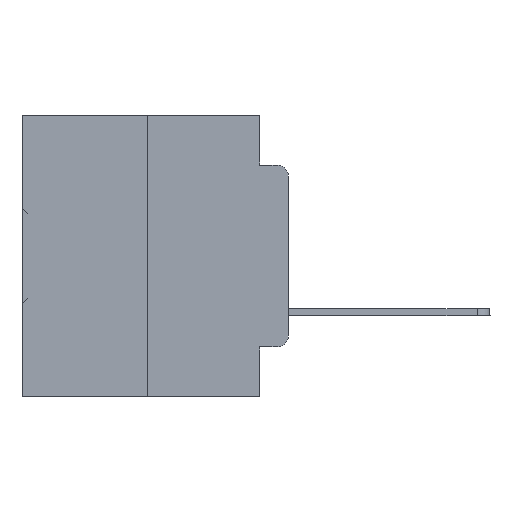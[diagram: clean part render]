
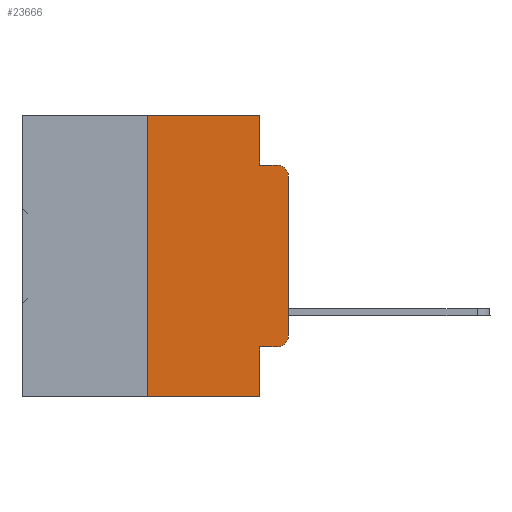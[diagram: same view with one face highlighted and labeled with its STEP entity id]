
A CAD part, left-side view. The second image highlights one B-rep face of the part: STEP entity #23666.
In plain terms, the highlighted planar face has unit normal (-1, 0, 0).
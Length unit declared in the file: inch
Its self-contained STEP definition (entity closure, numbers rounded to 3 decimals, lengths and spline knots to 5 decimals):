
#440 = CARTESIAN_POINT ( 'NONE',  ( 0., 0.25, 0. ) ) ;
#1844 = ORIENTED_EDGE ( 'NONE', *, *, #35728, .F. ) ;
#1858 = CARTESIAN_POINT ( 'NONE',  ( 0., 0.051, -0.0885 ) ) ;
#1861 = VERTEX_POINT ( 'NONE', #27456 ) ;
#2323 = CARTESIAN_POINT ( 'NONE',  ( 0., 0., -0.3915 ) ) ;
#2589 = DIRECTION ( 'NONE',  ( 0., 0., 1. ) ) ;
#2970 = EDGE_LOOP ( 'NONE', ( #31166, #35959, #24274, #21436, #34264, #14119, #27067, #1844, #8070, #9068 ) ) ;
#3821 = AXIS2_PLACEMENT_3D ( 'NONE', #16597, #28129, #8320 ) ;
#4102 = VECTOR ( 'NONE', #35673, 39.37008 ) ;
#4434 = EDGE_CURVE ( 'NONE', #31524, #20367, #23377, .T. ) ;
#4516 = FACE_OUTER_BOUND ( 'NONE', #2970, .T. ) ;
#4944 = CARTESIAN_POINT ( 'NONE',  ( 0., 0.051, -0.0885 ) ) ;
#4979 = AXIS2_PLACEMENT_3D ( 'NONE', #27903, #11076, #25078 ) ;
#5145 = VERTEX_POINT ( 'NONE', #29237 ) ;
#6379 = VERTEX_POINT ( 'NONE', #17656 ) ;
#6495 = LINE ( 'NONE', #20571, #27211 ) ;
#6740 = LINE ( 'NONE', #7071, #22135 ) ;
#7071 = CARTESIAN_POINT ( 'NONE',  ( 0., 0.051, 0. ) ) ;
#7100 = CARTESIAN_POINT ( 'NONE',  ( 0., 0.473, -0.5 ) ) ;
#8070 = ORIENTED_EDGE ( 'NONE', *, *, #13302, .T. ) ;
#8320 = DIRECTION ( 'NONE',  ( 0., 0., -1. ) ) ;
#9068 = ORIENTED_EDGE ( 'NONE', *, *, #19667, .T. ) ;
#9820 = LINE ( 'NONE', #29593, #4102 ) ;
#10162 = EDGE_CURVE ( 'NONE', #20367, #12212, #17248, .T. ) ;
#10170 = VECTOR ( 'NONE', #23088, 39.37008 ) ;
#10440 = EDGE_CURVE ( 'NONE', #30002, #5145, #31272, .T. ) ;
#10610 = CARTESIAN_POINT ( 'NONE',  ( 0., 0.051, 0. ) ) ;
#11076 = DIRECTION ( 'NONE',  ( -1., 0., 0. ) ) ;
#12212 = VERTEX_POINT ( 'NONE', #33256 ) ;
#12769 = DIRECTION ( 'NONE',  ( 0., -1., 0. ) ) ;
#13302 = EDGE_CURVE ( 'NONE', #1861, #6379, #6495, .T. ) ;
#13354 = DIRECTION ( 'NONE',  ( 0., 0., -1. ) ) ;
#13934 = AXIS2_PLACEMENT_3D ( 'NONE', #27362, #30185, #13354 ) ;
#14085 = VERTEX_POINT ( 'NONE', #4944 ) ;
#14119 = ORIENTED_EDGE ( 'NONE', *, *, #29017, .F. ) ;
#15822 = VERTEX_POINT ( 'NONE', #10610 ) ;
#16597 = CARTESIAN_POINT ( 'NONE',  ( 0., 0.02, -0.1085 ) ) ;
#17248 = CIRCLE ( 'NONE', #3821, 0.02 ) ;
#17330 = VECTOR ( 'NONE', #30160, 39.37008 ) ;
#17656 = CARTESIAN_POINT ( 'NONE',  ( 0., 0.02, -0.4115 ) ) ;
#18088 = LINE ( 'NONE', #440, #10170 ) ;
#18162 = CARTESIAN_POINT ( 'NONE',  ( 0., 0.051, 0. ) ) ;
#18804 = LINE ( 'NONE', #18162, #31080 ) ;
#19304 = DIRECTION ( 'NONE',  ( 0., -1., 0. ) ) ;
#19667 = EDGE_CURVE ( 'NONE', #6379, #31524, #30894, .T. ) ;
#20346 = EDGE_CURVE ( 'NONE', #15822, #14085, #18804, .T. ) ;
#20367 = VERTEX_POINT ( 'NONE', #26296 ) ;
#20571 = CARTESIAN_POINT ( 'NONE',  ( 0., 0.051, -0.4115 ) ) ;
#21436 = ORIENTED_EDGE ( 'NONE', *, *, #20346, .F. ) ;
#22052 = VERTEX_POINT ( 'NONE', #35470 ) ;
#22135 = VECTOR ( 'NONE', #29723, 39.37008 ) ;
#22176 = LINE ( 'NONE', #1858, #17330 ) ;
#22651 = EDGE_CURVE ( 'NONE', #14085, #12212, #22176, .T. ) ;
#22879 = EDGE_CURVE ( 'NONE', #22052, #15822, #9820, .T. ) ;
#23088 = DIRECTION ( 'NONE',  ( 0., 0., 1. ) ) ;
#23377 = LINE ( 'NONE', #33424, #34351 ) ;
#23666 = ADVANCED_FACE ( 'NONE', ( #4516 ), #32873, .F. ) ;
#24274 = ORIENTED_EDGE ( 'NONE', *, *, #22651, .F. ) ;
#25078 = DIRECTION ( 'NONE',  ( 0., 0., -1. ) ) ;
#26296 = CARTESIAN_POINT ( 'NONE',  ( 0., 0., -0.1085 ) ) ;
#26441 = VECTOR ( 'NONE', #12769, 39.37008 ) ;
#27067 = ORIENTED_EDGE ( 'NONE', *, *, #10440, .T. ) ;
#27211 = VECTOR ( 'NONE', #19304, 39.37008 ) ;
#27362 = CARTESIAN_POINT ( 'NONE',  ( 0., 0.473, 0. ) ) ;
#27456 = CARTESIAN_POINT ( 'NONE',  ( 0., 0.051, -0.4115 ) ) ;
#27903 = CARTESIAN_POINT ( 'NONE',  ( 0., 0.02, -0.3915 ) ) ;
#28129 = DIRECTION ( 'NONE',  ( -1., 0., 0. ) ) ;
#28298 = DIRECTION ( 'NONE',  ( 0., 0., -1. ) ) ;
#29017 = EDGE_CURVE ( 'NONE', #30002, #22052, #18088, .T. ) ;
#29237 = CARTESIAN_POINT ( 'NONE',  ( 0., 0.051, -0.5 ) ) ;
#29593 = CARTESIAN_POINT ( 'NONE',  ( 0., 0.473, 0. ) ) ;
#29723 = DIRECTION ( 'NONE',  ( 0., 0., -1. ) ) ;
#30002 = VERTEX_POINT ( 'NONE', #33026 ) ;
#30160 = DIRECTION ( 'NONE',  ( 0., -1., 0. ) ) ;
#30185 = DIRECTION ( 'NONE',  ( 1., 0., 0. ) ) ;
#30894 = CIRCLE ( 'NONE', #4979, 0.02 ) ;
#31080 = VECTOR ( 'NONE', #28298, 39.37008 ) ;
#31166 = ORIENTED_EDGE ( 'NONE', *, *, #4434, .T. ) ;
#31272 = LINE ( 'NONE', #7100, #26441 ) ;
#31524 = VERTEX_POINT ( 'NONE', #2323 ) ;
#32873 = PLANE ( 'NONE',  #13934 ) ;
#33026 = CARTESIAN_POINT ( 'NONE',  ( 0., 0.25, -0.5 ) ) ;
#33256 = CARTESIAN_POINT ( 'NONE',  ( 0., 0.02, -0.0885 ) ) ;
#33424 = CARTESIAN_POINT ( 'NONE',  ( 0., 0., 0. ) ) ;
#34264 = ORIENTED_EDGE ( 'NONE', *, *, #22879, .F. ) ;
#34351 = VECTOR ( 'NONE', #2589, 39.37008 ) ;
#35470 = CARTESIAN_POINT ( 'NONE',  ( 0., 0.25, 0. ) ) ;
#35673 = DIRECTION ( 'NONE',  ( 0., -1., 0. ) ) ;
#35728 = EDGE_CURVE ( 'NONE', #1861, #5145, #6740, .T. ) ;
#35959 = ORIENTED_EDGE ( 'NONE', *, *, #10162, .T. ) ;
